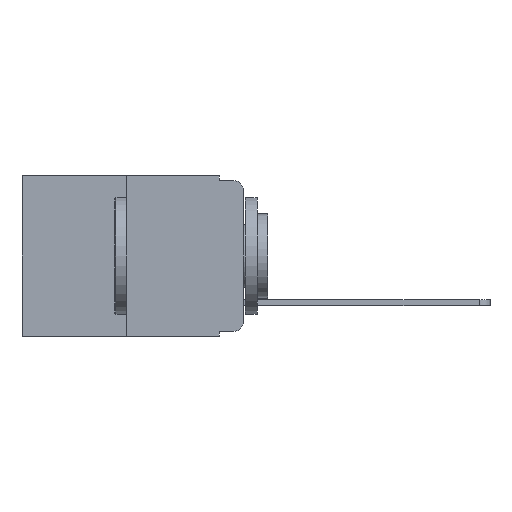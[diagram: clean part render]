
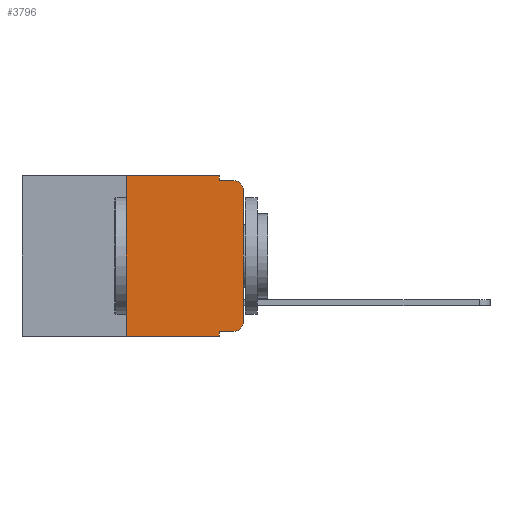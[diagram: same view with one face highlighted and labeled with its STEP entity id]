
A CAD part, left-side view. The second image highlights one B-rep face of the part: STEP entity #3796.
In plain terms, the highlighted planar face has unit normal (-1, 0, 0).
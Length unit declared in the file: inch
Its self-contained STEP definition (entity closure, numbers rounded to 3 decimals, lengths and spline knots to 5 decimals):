
#122 = ORIENTED_EDGE ( 'NONE', *, *, #4983, .F. ) ;
#219 = DIRECTION ( 'NONE',  ( -1., 0., 0. ) ) ;
#345 = PLANE ( 'NONE',  #6038 ) ;
#486 = DIRECTION ( 'NONE',  ( 0., -1., 0. ) ) ;
#658 = AXIS2_PLACEMENT_3D ( 'NONE', #5592, #219, #6445 ) ;
#973 = VERTEX_POINT ( 'NONE', #4067 ) ;
#1190 = VECTOR ( 'NONE', #9976, 39.37008 ) ;
#1338 = VECTOR ( 'NONE', #2528, 39.37008 ) ;
#1365 = VERTEX_POINT ( 'NONE', #4174 ) ;
#1772 = DIRECTION ( 'NONE',  ( 0., -1., 0. ) ) ;
#2019 = EDGE_CURVE ( 'NONE', #2082, #10718, #9367, .T. ) ;
#2022 = ORIENTED_EDGE ( 'NONE', *, *, #2019, .F. ) ;
#2047 = ORIENTED_EDGE ( 'NONE', *, *, #3237, .F. ) ;
#2066 = DIRECTION ( 'NONE',  ( 0., 0., -1. ) ) ;
#2082 = VERTEX_POINT ( 'NONE', #9277 ) ;
#2528 = DIRECTION ( 'NONE',  ( 0., 0., -1. ) ) ;
#2559 = DIRECTION ( 'NONE',  ( 0., -1., 0. ) ) ;
#2961 = CARTESIAN_POINT ( 'NONE',  ( 0., 0.051, 0. ) ) ;
#2998 = VERTEX_POINT ( 'NONE', #4811 ) ;
#3207 = VECTOR ( 'NONE', #1772, 39.37008 ) ;
#3237 = EDGE_CURVE ( 'NONE', #3872, #10846, #8455, .T. ) ;
#3318 = EDGE_CURVE ( 'NONE', #3872, #10718, #6453, .T. ) ;
#3471 = ORIENTED_EDGE ( 'NONE', *, *, #4758, .T. ) ;
#3796 = ADVANCED_FACE ( 'NONE', ( #6726 ), #345, .F. ) ;
#3872 = VERTEX_POINT ( 'NONE', #4561 ) ;
#3972 = DIRECTION ( 'NONE',  ( 1., 0., 0. ) ) ;
#4067 = CARTESIAN_POINT ( 'NONE',  ( 0., 0., -0.03 ) ) ;
#4174 = CARTESIAN_POINT ( 'NONE',  ( 0., 0., -0.313 ) ) ;
#4236 = ORIENTED_EDGE ( 'NONE', *, *, #8968, .F. ) ;
#4561 = CARTESIAN_POINT ( 'NONE',  ( 0., 0.25, -0.343 ) ) ;
#4758 = EDGE_CURVE ( 'NONE', #1365, #973, #5928, .T. ) ;
#4811 = CARTESIAN_POINT ( 'NONE',  ( 0., 0.02, -0.333 ) ) ;
#4888 = CIRCLE ( 'NONE', #10749, 0.02 ) ;
#4939 = CARTESIAN_POINT ( 'NONE',  ( 0., 0.051, 0. ) ) ;
#4983 = EDGE_CURVE ( 'NONE', #5749, #5232, #8291, .T. ) ;
#5025 = ORIENTED_EDGE ( 'NONE', *, *, #8048, .T. ) ;
#5069 = ORIENTED_EDGE ( 'NONE', *, *, #6122, .F. ) ;
#5232 = VERTEX_POINT ( 'NONE', #8221 ) ;
#5300 = ORIENTED_EDGE ( 'NONE', *, *, #6344, .T. ) ;
#5347 = CARTESIAN_POINT ( 'NONE',  ( 0., 0.02, -0.03 ) ) ;
#5500 = CARTESIAN_POINT ( 'NONE',  ( 0., 0.473, -0.343 ) ) ;
#5519 = DIRECTION ( 'NONE',  ( 0., 0., 1. ) ) ;
#5592 = CARTESIAN_POINT ( 'NONE',  ( 0., 0.02, -0.313 ) ) ;
#5749 = VERTEX_POINT ( 'NONE', #2961 ) ;
#5928 = LINE ( 'NONE', #10128, #1190 ) ;
#6009 = ORIENTED_EDGE ( 'NONE', *, *, #11159, .T. ) ;
#6038 = AXIS2_PLACEMENT_3D ( 'NONE', #6700, #3972, #2066 ) ;
#6122 = EDGE_CURVE ( 'NONE', #10846, #5749, #9985, .T. ) ;
#6220 = DIRECTION ( 'NONE',  ( 0., 0., -1. ) ) ;
#6296 = LINE ( 'NONE', #6695, #8284 ) ;
#6344 = EDGE_CURVE ( 'NONE', #2998, #1365, #7365, .T. ) ;
#6362 = DIRECTION ( 'NONE',  ( 0., 0., -1. ) ) ;
#6444 = CARTESIAN_POINT ( 'NONE',  ( 0., 0.051, -0.343 ) ) ;
#6445 = DIRECTION ( 'NONE',  ( 0., 0., -1. ) ) ;
#6453 = LINE ( 'NONE', #5500, #9853 ) ;
#6695 = CARTESIAN_POINT ( 'NONE',  ( 0., 0.051, -0.01 ) ) ;
#6700 = CARTESIAN_POINT ( 'NONE',  ( 0., 0.473, 0. ) ) ;
#6715 = DIRECTION ( 'NONE',  ( 0., -1., 0. ) ) ;
#6726 = FACE_OUTER_BOUND ( 'NONE', #7051, .T. ) ;
#7015 = CARTESIAN_POINT ( 'NONE',  ( 0., 0.473, 0. ) ) ;
#7051 = EDGE_LOOP ( 'NONE', ( #3471, #6009, #4236, #122, #5069, #2047, #8931, #2022, #5025, #5300 ) ) ;
#7316 = CARTESIAN_POINT ( 'NONE',  ( 0., 0.02, -0.01 ) ) ;
#7365 = CIRCLE ( 'NONE', #658, 0.02 ) ;
#7404 = VECTOR ( 'NONE', #6362, 39.37008 ) ;
#7727 = CARTESIAN_POINT ( 'NONE',  ( 0., 0.051, -0.333 ) ) ;
#7902 = VERTEX_POINT ( 'NONE', #7316 ) ;
#8048 = EDGE_CURVE ( 'NONE', #2082, #2998, #10080, .T. ) ;
#8221 = CARTESIAN_POINT ( 'NONE',  ( 0., 0.051, -0.01 ) ) ;
#8284 = VECTOR ( 'NONE', #486, 39.37008 ) ;
#8291 = LINE ( 'NONE', #4939, #1338 ) ;
#8455 = LINE ( 'NONE', #8526, #8718 ) ;
#8526 = CARTESIAN_POINT ( 'NONE',  ( 0., 0.25, 0. ) ) ;
#8718 = VECTOR ( 'NONE', #5519, 39.37008 ) ;
#8931 = ORIENTED_EDGE ( 'NONE', *, *, #3318, .T. ) ;
#8968 = EDGE_CURVE ( 'NONE', #5232, #7902, #6296, .T. ) ;
#9261 = CARTESIAN_POINT ( 'NONE',  ( 0., 0.051, 0. ) ) ;
#9277 = CARTESIAN_POINT ( 'NONE',  ( 0., 0.051, -0.333 ) ) ;
#9367 = LINE ( 'NONE', #9261, #7404 ) ;
#9853 = VECTOR ( 'NONE', #6715, 39.37008 ) ;
#9976 = DIRECTION ( 'NONE',  ( 0., 0., 1. ) ) ;
#9985 = LINE ( 'NONE', #7015, #3207 ) ;
#10080 = LINE ( 'NONE', #7727, #10340 ) ;
#10128 = CARTESIAN_POINT ( 'NONE',  ( 0., 0., 0. ) ) ;
#10340 = VECTOR ( 'NONE', #2559, 39.37008 ) ;
#10718 = VERTEX_POINT ( 'NONE', #6444 ) ;
#10749 = AXIS2_PLACEMENT_3D ( 'NONE', #5347, #11197, #6220 ) ;
#10785 = CARTESIAN_POINT ( 'NONE',  ( 0., 0.25, 0. ) ) ;
#10846 = VERTEX_POINT ( 'NONE', #10785 ) ;
#11159 = EDGE_CURVE ( 'NONE', #973, #7902, #4888, .T. ) ;
#11197 = DIRECTION ( 'NONE',  ( -1., 0., 0. ) ) ;
